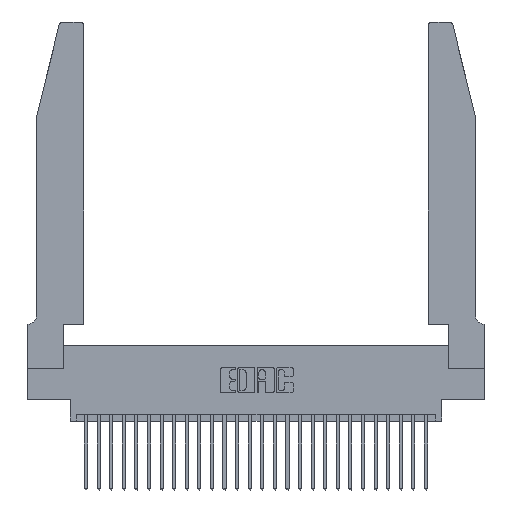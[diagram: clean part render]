
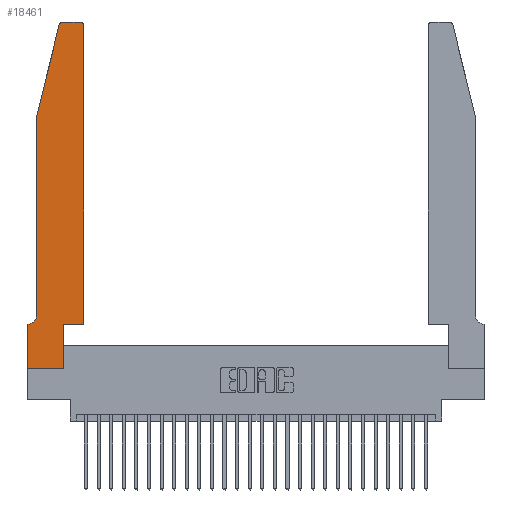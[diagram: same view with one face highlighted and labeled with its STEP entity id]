
A CAD part, top view. The second image highlights one B-rep face of the part: STEP entity #18461.
In plain terms, the highlighted planar face has unit normal (0, 0, 1).
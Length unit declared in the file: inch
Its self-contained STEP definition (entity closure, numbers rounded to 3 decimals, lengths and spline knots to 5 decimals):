
#88 = VECTOR ( 'NONE', #26852, 39.37008 ) ;
#383 = EDGE_CURVE ( 'NONE', #27245, #7709, #2285, .T. ) ;
#694 = VERTEX_POINT ( 'NONE', #26666 ) ;
#796 = ORIENTED_EDGE ( 'NONE', *, *, #4102, .T. ) ;
#877 = LINE ( 'NONE', #28142, #12332 ) ;
#907 = VERTEX_POINT ( 'NONE', #26183 ) ;
#997 = ORIENTED_EDGE ( 'NONE', *, *, #383, .T. ) ;
#1046 = DIRECTION ( 'NONE',  ( 0., 1., 0. ) ) ;
#1188 = DIRECTION ( 'NONE',  ( -1., 0., 0. ) ) ;
#1782 = EDGE_CURVE ( 'NONE', #22935, #10247, #15916, .T. ) ;
#1916 = DIRECTION ( 'NONE',  ( -1., 0., 0. ) ) ;
#2005 = CARTESIAN_POINT ( 'NONE',  ( 0.2605, 2.75, 0.37 ) ) ;
#2249 = AXIS2_PLACEMENT_3D ( 'NONE', #27590, #3330, #7361 ) ;
#2285 = CIRCLE ( 'NONE', #2249, 0.07 ) ;
#2415 = CARTESIAN_POINT ( 'NONE',  ( 0., 0.35, 0.37 ) ) ;
#2614 = DIRECTION ( 'NONE',  ( 0., 0., 1. ) ) ;
#3285 = CARTESIAN_POINT ( 'NONE',  ( 0.0755, 0.42, 0.37 ) ) ;
#3330 = DIRECTION ( 'NONE',  ( 0., 0., -1. ) ) ;
#3633 = VERTEX_POINT ( 'NONE', #22479 ) ;
#3751 = ORIENTED_EDGE ( 'NONE', *, *, #22899, .T. ) ;
#3923 = ORIENTED_EDGE ( 'NONE', *, *, #15686, .T. ) ;
#4102 = EDGE_CURVE ( 'NONE', #4510, #27245, #877, .T. ) ;
#4510 = VERTEX_POINT ( 'NONE', #10089 ) ;
#4770 = CIRCLE ( 'NONE', #8307, 0.03 ) ;
#4881 = VERTEX_POINT ( 'NONE', #11156 ) ;
#5477 = CARTESIAN_POINT ( 'NONE',  ( 0.2865, 0., 0.37 ) ) ;
#5508 = DIRECTION ( 'NONE',  ( 1., 0., 0. ) ) ;
#5649 = EDGE_CURVE ( 'NONE', #4881, #22935, #4770, .T. ) ;
#6969 = ORIENTED_EDGE ( 'NONE', *, *, #7332, .T. ) ;
#7010 = CARTESIAN_POINT ( 'NONE',  ( 0.0755, 2., 0.37 ) ) ;
#7155 = DIRECTION ( 'NONE',  ( 0., 0., 1. ) ) ;
#7332 = EDGE_CURVE ( 'NONE', #694, #3633, #8980, .T. ) ;
#7361 = DIRECTION ( 'NONE',  ( -1., 0., 0. ) ) ;
#7400 = EDGE_LOOP ( 'NONE', ( #7860, #3751, #21459, #796, #997, #14714, #11343, #22347, #23367, #6969, #3923, #27073 ) ) ;
#7709 = VERTEX_POINT ( 'NONE', #24568 ) ;
#7723 = EDGE_CURVE ( 'NONE', #907, #4510, #28437, .T. ) ;
#7810 = VECTOR ( 'NONE', #1188, 39.37008 ) ;
#7860 = ORIENTED_EDGE ( 'NONE', *, *, #1782, .T. ) ;
#8166 = LINE ( 'NONE', #13199, #19317 ) ;
#8266 = VECTOR ( 'NONE', #5508, 39.37008 ) ;
#8307 = AXIS2_PLACEMENT_3D ( 'NONE', #22156, #8898, #24290 ) ;
#8571 = DIRECTION ( 'NONE',  ( 1., 0., 0. ) ) ;
#8898 = DIRECTION ( 'NONE',  ( 0., 0., 1. ) ) ;
#8980 = LINE ( 'NONE', #23199, #8266 ) ;
#9036 = EDGE_CURVE ( 'NONE', #7709, #15704, #14490, .T. ) ;
#9441 = CARTESIAN_POINT ( 'NONE',  ( 0., 0.35, 0.37 ) ) ;
#10079 = CARTESIAN_POINT ( 'NONE',  ( 0.2865, 0.35, 0.37 ) ) ;
#10089 = CARTESIAN_POINT ( 'NONE',  ( 0.0755, 2., 0.37 ) ) ;
#10247 = VERTEX_POINT ( 'NONE', #12039 ) ;
#11156 = CARTESIAN_POINT ( 'NONE',  ( 0.4505, 2.72, 0.37 ) ) ;
#11343 = ORIENTED_EDGE ( 'NONE', *, *, #24034, .T. ) ;
#11619 = CARTESIAN_POINT ( 'NONE',  ( 0.4505, 0.35, 0.37 ) ) ;
#12039 = CARTESIAN_POINT ( 'NONE',  ( 0.284, 2.75, 0.37 ) ) ;
#12332 = VECTOR ( 'NONE', #17444, 39.37008 ) ;
#12581 = CARTESIAN_POINT ( 'NONE',  ( 0.0755, 0.35, 0.37 ) ) ;
#13199 = CARTESIAN_POINT ( 'NONE',  ( 0., 0., 0.37 ) ) ;
#13936 = EDGE_CURVE ( 'NONE', #21769, #694, #14130, .T. ) ;
#13989 = VERTEX_POINT ( 'NONE', #14867 ) ;
#14130 = LINE ( 'NONE', #10079, #23675 ) ;
#14490 = LINE ( 'NONE', #12581, #7810 ) ;
#14499 = VECTOR ( 'NONE', #1916, 39.37008 ) ;
#14714 = ORIENTED_EDGE ( 'NONE', *, *, #9036, .T. ) ;
#14867 = CARTESIAN_POINT ( 'NONE',  ( 0., 0., 0.37 ) ) ;
#15112 = AXIS2_PLACEMENT_3D ( 'NONE', #2415, #2614, #18413 ) ;
#15686 = EDGE_CURVE ( 'NONE', #3633, #4881, #17504, .T. ) ;
#15704 = VERTEX_POINT ( 'NONE', #9441 ) ;
#15916 = LINE ( 'NONE', #2005, #14499 ) ;
#16211 = PLANE ( 'NONE',  #15112 ) ;
#16641 = VECTOR ( 'NONE', #27251, 39.37008 ) ;
#17014 = VECTOR ( 'NONE', #24665, 39.37008 ) ;
#17444 = DIRECTION ( 'NONE',  ( 0., -1., 0. ) ) ;
#17504 = LINE ( 'NONE', #11619, #88 ) ;
#18402 = CIRCLE ( 'NONE', #24944, 0.03 ) ;
#18413 = DIRECTION ( 'NONE',  ( 1., 0., 0. ) ) ;
#18461 = ADVANCED_FACE ( 'NONE', ( #24810 ), #16211, .T. ) ;
#19317 = VECTOR ( 'NONE', #8571, 39.37008 ) ;
#20502 = CARTESIAN_POINT ( 'NONE',  ( 0.284, 2.72, 0.37 ) ) ;
#20592 = CARTESIAN_POINT ( 'NONE',  ( 0.4205, 2.75, 0.37 ) ) ;
#21459 = ORIENTED_EDGE ( 'NONE', *, *, #7723, .T. ) ;
#21769 = VERTEX_POINT ( 'NONE', #5477 ) ;
#22156 = CARTESIAN_POINT ( 'NONE',  ( 0.4205, 2.72, 0.37 ) ) ;
#22347 = ORIENTED_EDGE ( 'NONE', *, *, #24356, .T. ) ;
#22389 = LINE ( 'NONE', #25132, #16641 ) ;
#22479 = CARTESIAN_POINT ( 'NONE',  ( 0.4505, 0.35, 0.37 ) ) ;
#22667 = DIRECTION ( 'NONE',  ( 1., 0., 0. ) ) ;
#22899 = EDGE_CURVE ( 'NONE', #10247, #907, #18402, .T. ) ;
#22935 = VERTEX_POINT ( 'NONE', #20592 ) ;
#23199 = CARTESIAN_POINT ( 'NONE',  ( 0.4505, 0.35, 0.37 ) ) ;
#23367 = ORIENTED_EDGE ( 'NONE', *, *, #13936, .T. ) ;
#23675 = VECTOR ( 'NONE', #1046, 39.37008 ) ;
#24034 = EDGE_CURVE ( 'NONE', #15704, #13989, #22389, .T. ) ;
#24290 = DIRECTION ( 'NONE',  ( 1., 0., 0. ) ) ;
#24356 = EDGE_CURVE ( 'NONE', #13989, #21769, #8166, .T. ) ;
#24568 = CARTESIAN_POINT ( 'NONE',  ( 0.0055, 0.35, 0.37 ) ) ;
#24665 = DIRECTION ( 'NONE',  ( -0.239, -0.971, 0. ) ) ;
#24810 = FACE_OUTER_BOUND ( 'NONE', #7400, .T. ) ;
#24944 = AXIS2_PLACEMENT_3D ( 'NONE', #20502, #7155, #22667 ) ;
#25132 = CARTESIAN_POINT ( 'NONE',  ( 0., 0., 0.37 ) ) ;
#26183 = CARTESIAN_POINT ( 'NONE',  ( 0.25487, 2.72718, 0.37 ) ) ;
#26666 = CARTESIAN_POINT ( 'NONE',  ( 0.2865, 0.35, 0.37 ) ) ;
#26852 = DIRECTION ( 'NONE',  ( 0., 1., 0. ) ) ;
#27073 = ORIENTED_EDGE ( 'NONE', *, *, #5649, .T. ) ;
#27245 = VERTEX_POINT ( 'NONE', #3285 ) ;
#27251 = DIRECTION ( 'NONE',  ( 0., -1., 0. ) ) ;
#27590 = CARTESIAN_POINT ( 'NONE',  ( 0.0055, 0.42, 0.37 ) ) ;
#28142 = CARTESIAN_POINT ( 'NONE',  ( 0.0755, 2., 0.37 ) ) ;
#28437 = LINE ( 'NONE', #7010, #17014 ) ;
